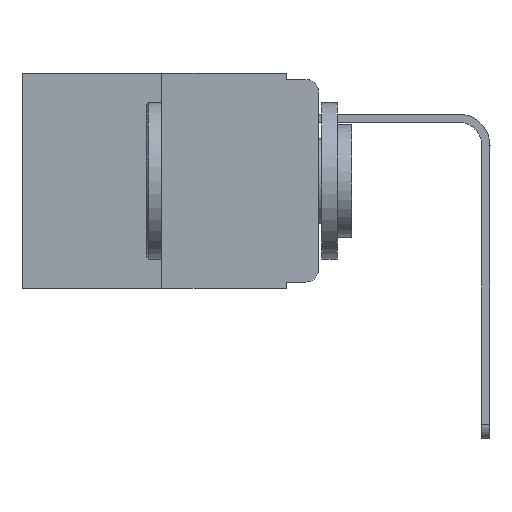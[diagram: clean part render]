
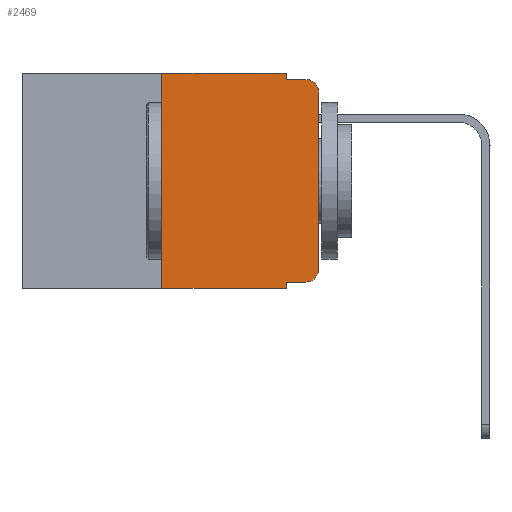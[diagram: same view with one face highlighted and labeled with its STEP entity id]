
A CAD part, left-side view. The second image highlights one B-rep face of the part: STEP entity #2469.
In plain terms, the highlighted planar face has unit normal (-1, 0, 0).
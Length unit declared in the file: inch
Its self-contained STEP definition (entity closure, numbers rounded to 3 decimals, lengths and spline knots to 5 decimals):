
#319 = CIRCLE ( 'NONE', #14453, 0.02 ) ;
#425 = LINE ( 'NONE', #5745, #4425 ) ;
#655 = VERTEX_POINT ( 'NONE', #10835 ) ;
#1006 = LINE ( 'NONE', #10159, #10446 ) ;
#1264 = VERTEX_POINT ( 'NONE', #11769 ) ;
#1483 = AXIS2_PLACEMENT_3D ( 'NONE', #12921, #8309, #15796 ) ;
#1503 = DIRECTION ( 'NONE',  ( 0., 0., -1. ) ) ;
#1550 = VERTEX_POINT ( 'NONE', #13119 ) ;
#1594 = LINE ( 'NONE', #11825, #10749 ) ;
#2469 = ADVANCED_FACE ( 'NONE', ( #11144 ), #17580, .F. ) ;
#3000 = VERTEX_POINT ( 'NONE', #8248 ) ;
#3654 = LINE ( 'NONE', #4567, #18339 ) ;
#4182 = ORIENTED_EDGE ( 'NONE', *, *, #7217, .T. ) ;
#4192 = DIRECTION ( 'NONE',  ( 0., -1., 0. ) ) ;
#4425 = VECTOR ( 'NONE', #16339, 39.37008 ) ;
#4470 = EDGE_CURVE ( 'NONE', #655, #16679, #16075, .T. ) ;
#4567 = CARTESIAN_POINT ( 'NONE',  ( 0., 0.051, 0. ) ) ;
#5202 = EDGE_CURVE ( 'NONE', #3000, #1550, #3654, .T. ) ;
#5745 = CARTESIAN_POINT ( 'NONE',  ( 0., 0.051, 0. ) ) ;
#6019 = AXIS2_PLACEMENT_3D ( 'NONE', #6533, #9837, #17137 ) ;
#6354 = VERTEX_POINT ( 'NONE', #16628 ) ;
#6533 = CARTESIAN_POINT ( 'NONE',  ( 0., 0.02, -0.03 ) ) ;
#7217 = EDGE_CURVE ( 'NONE', #13996, #655, #319, .T. ) ;
#7233 = ORIENTED_EDGE ( 'NONE', *, *, #9432, .T. ) ;
#7260 = ORIENTED_EDGE ( 'NONE', *, *, #15278, .F. ) ;
#7656 = EDGE_CURVE ( 'NONE', #1264, #3000, #7843, .T. ) ;
#7804 = EDGE_LOOP ( 'NONE', ( #10145, #7233, #18610, #12365, #9761, #7260, #11136, #9725, #12595, #4182 ) ) ;
#7843 = LINE ( 'NONE', #8944, #11846 ) ;
#7857 = LINE ( 'NONE', #18174, #11621 ) ;
#8248 = CARTESIAN_POINT ( 'NONE',  ( 0., 0.051, 0. ) ) ;
#8309 = DIRECTION ( 'NONE',  ( 1., 0., 0. ) ) ;
#8568 = CARTESIAN_POINT ( 'NONE',  ( 0., 0.02, -0.313 ) ) ;
#8944 = CARTESIAN_POINT ( 'NONE',  ( 0., 0.473, 0. ) ) ;
#9432 = EDGE_CURVE ( 'NONE', #16679, #17696, #10595, .T. ) ;
#9725 = ORIENTED_EDGE ( 'NONE', *, *, #18957, .F. ) ;
#9761 = ORIENTED_EDGE ( 'NONE', *, *, #7656, .F. ) ;
#9837 = DIRECTION ( 'NONE',  ( -1., 0., 0. ) ) ;
#10084 = EDGE_CURVE ( 'NONE', #6354, #13996, #12925, .T. ) ;
#10112 = VECTOR ( 'NONE', #13618, 39.37008 ) ;
#10143 = DIRECTION ( 'NONE',  ( -1., 0., 0. ) ) ;
#10145 = ORIENTED_EDGE ( 'NONE', *, *, #4470, .T. ) ;
#10159 = CARTESIAN_POINT ( 'NONE',  ( 0., 0.25, 0. ) ) ;
#10446 = VECTOR ( 'NONE', #11672, 39.37008 ) ;
#10595 = CIRCLE ( 'NONE', #6019, 0.02 ) ;
#10749 = VECTOR ( 'NONE', #4192, 39.37008 ) ;
#10835 = CARTESIAN_POINT ( 'NONE',  ( 0., 0., -0.313 ) ) ;
#11066 = CARTESIAN_POINT ( 'NONE',  ( 0., 0.25, -0.343 ) ) ;
#11136 = ORIENTED_EDGE ( 'NONE', *, *, #14317, .T. ) ;
#11144 = FACE_OUTER_BOUND ( 'NONE', #7804, .T. ) ;
#11185 = CARTESIAN_POINT ( 'NONE',  ( 0., 0.02, -0.333 ) ) ;
#11525 = VERTEX_POINT ( 'NONE', #16937 ) ;
#11565 = VERTEX_POINT ( 'NONE', #11066 ) ;
#11621 = VECTOR ( 'NONE', #17089, 39.37008 ) ;
#11672 = DIRECTION ( 'NONE',  ( 0., 0., 1. ) ) ;
#11769 = CARTESIAN_POINT ( 'NONE',  ( 0., 0.25, 0. ) ) ;
#11825 = CARTESIAN_POINT ( 'NONE',  ( 0., 0.051, -0.01 ) ) ;
#11846 = VECTOR ( 'NONE', #16552, 39.37008 ) ;
#12222 = CARTESIAN_POINT ( 'NONE',  ( 0., 0., 0. ) ) ;
#12365 = ORIENTED_EDGE ( 'NONE', *, *, #5202, .F. ) ;
#12435 = CARTESIAN_POINT ( 'NONE',  ( 0., 0.02, -0.01 ) ) ;
#12595 = ORIENTED_EDGE ( 'NONE', *, *, #10084, .T. ) ;
#12800 = EDGE_CURVE ( 'NONE', #1550, #17696, #1594, .T. ) ;
#12861 = CARTESIAN_POINT ( 'NONE',  ( 0., 0., -0.03 ) ) ;
#12921 = CARTESIAN_POINT ( 'NONE',  ( 0., 0.473, 0. ) ) ;
#12925 = LINE ( 'NONE', #16796, #10112 ) ;
#13119 = CARTESIAN_POINT ( 'NONE',  ( 0., 0.051, -0.01 ) ) ;
#13618 = DIRECTION ( 'NONE',  ( 0., -1., 0. ) ) ;
#13996 = VERTEX_POINT ( 'NONE', #11185 ) ;
#14317 = EDGE_CURVE ( 'NONE', #11565, #11525, #7857, .T. ) ;
#14453 = AXIS2_PLACEMENT_3D ( 'NONE', #8568, #10143, #19364 ) ;
#14900 = VECTOR ( 'NONE', #19010, 39.37008 ) ;
#15278 = EDGE_CURVE ( 'NONE', #11565, #1264, #1006, .T. ) ;
#15796 = DIRECTION ( 'NONE',  ( 0., 0., -1. ) ) ;
#16075 = LINE ( 'NONE', #12222, #14900 ) ;
#16339 = DIRECTION ( 'NONE',  ( 0., 0., -1. ) ) ;
#16552 = DIRECTION ( 'NONE',  ( 0., -1., 0. ) ) ;
#16628 = CARTESIAN_POINT ( 'NONE',  ( 0., 0.051, -0.333 ) ) ;
#16679 = VERTEX_POINT ( 'NONE', #12861 ) ;
#16796 = CARTESIAN_POINT ( 'NONE',  ( 0., 0.051, -0.333 ) ) ;
#16937 = CARTESIAN_POINT ( 'NONE',  ( 0., 0.051, -0.343 ) ) ;
#17089 = DIRECTION ( 'NONE',  ( 0., -1., 0. ) ) ;
#17137 = DIRECTION ( 'NONE',  ( 0., 0., -1. ) ) ;
#17580 = PLANE ( 'NONE',  #1483 ) ;
#17696 = VERTEX_POINT ( 'NONE', #12435 ) ;
#18174 = CARTESIAN_POINT ( 'NONE',  ( 0., 0.473, -0.343 ) ) ;
#18339 = VECTOR ( 'NONE', #1503, 39.37008 ) ;
#18610 = ORIENTED_EDGE ( 'NONE', *, *, #12800, .F. ) ;
#18957 = EDGE_CURVE ( 'NONE', #6354, #11525, #425, .T. ) ;
#19010 = DIRECTION ( 'NONE',  ( 0., 0., 1. ) ) ;
#19364 = DIRECTION ( 'NONE',  ( 0., 0., -1. ) ) ;
